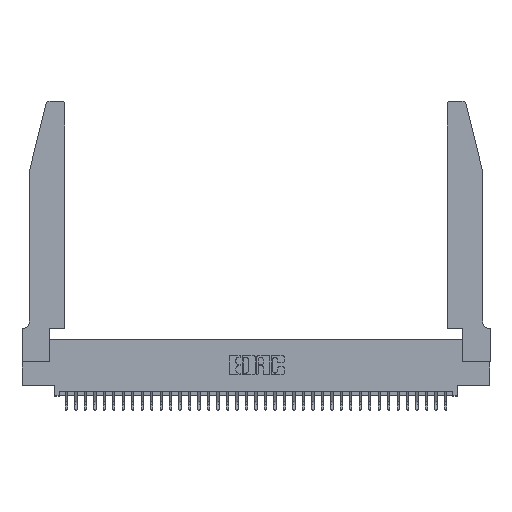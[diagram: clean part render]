
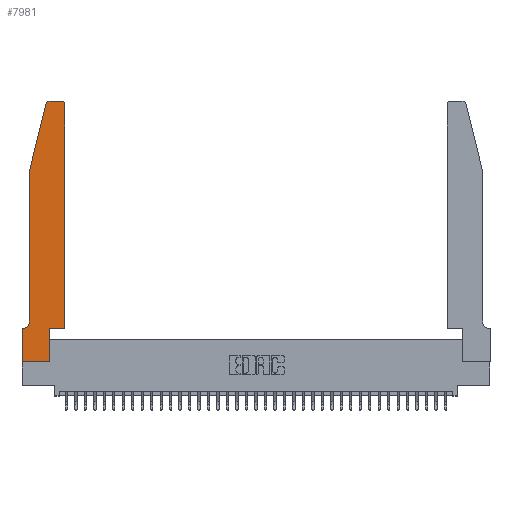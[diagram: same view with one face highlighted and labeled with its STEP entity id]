
A CAD part, top view. The second image highlights one B-rep face of the part: STEP entity #7981.
In plain terms, the highlighted planar face has unit normal (0, 0, 1).
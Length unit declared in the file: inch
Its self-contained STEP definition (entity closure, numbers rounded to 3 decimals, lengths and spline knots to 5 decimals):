
#51 = LINE ( 'NONE', #12348, #7271 ) ;
#1088 = DIRECTION ( 'NONE',  ( 0., -1., 0. ) ) ;
#2117 = EDGE_CURVE ( 'NONE', #23884, #32361, #51, .T. ) ;
#2524 = EDGE_CURVE ( 'NONE', #32361, #19270, #25403, .T. ) ;
#2597 = CARTESIAN_POINT ( 'NONE',  ( 0.4505, 0.35, 0.37 ) ) ;
#3032 = EDGE_CURVE ( 'NONE', #11793, #6742, #24887, .T. ) ;
#3141 = DIRECTION ( 'NONE',  ( -1., 0., 0. ) ) ;
#3197 = LINE ( 'NONE', #21606, #13162 ) ;
#3855 = VECTOR ( 'NONE', #11667, 39.37008 ) ;
#4039 = CARTESIAN_POINT ( 'NONE',  ( 0.284, 2.72, 0.37 ) ) ;
#4614 = VECTOR ( 'NONE', #3141, 39.37008 ) ;
#4789 = DIRECTION ( 'NONE',  ( -1., 0., 0. ) ) ;
#4888 = CARTESIAN_POINT ( 'NONE',  ( 0.284, 2.75, 0.37 ) ) ;
#6269 = ORIENTED_EDGE ( 'NONE', *, *, #2524, .T. ) ;
#6742 = VERTEX_POINT ( 'NONE', #8463 ) ;
#7030 = ORIENTED_EDGE ( 'NONE', *, *, #36220, .T. ) ;
#7140 = VERTEX_POINT ( 'NONE', #4888 ) ;
#7239 = VERTEX_POINT ( 'NONE', #24668 ) ;
#7271 = VECTOR ( 'NONE', #9415, 39.37008 ) ;
#7814 = AXIS2_PLACEMENT_3D ( 'NONE', #26194, #31943, #34428 ) ;
#7981 = ADVANCED_FACE ( 'NONE', ( #32245 ), #13651, .T. ) ;
#8097 = DIRECTION ( 'NONE',  ( 1., 0., 0. ) ) ;
#8406 = EDGE_CURVE ( 'NONE', #20728, #28738, #24589, .T. ) ;
#8463 = CARTESIAN_POINT ( 'NONE',  ( 0.0755, 2., 0.37 ) ) ;
#8531 = VERTEX_POINT ( 'NONE', #32707 ) ;
#9072 = VECTOR ( 'NONE', #34392, 39.37008 ) ;
#9250 = CARTESIAN_POINT ( 'NONE',  ( 0.0755, 2., 0.37 ) ) ;
#9415 = DIRECTION ( 'NONE',  ( 1., 0., 0. ) ) ;
#9711 = AXIS2_PLACEMENT_3D ( 'NONE', #4039, #15444, #15561 ) ;
#11203 = VERTEX_POINT ( 'NONE', #29097 ) ;
#11288 = CIRCLE ( 'NONE', #22662, 0.07 ) ;
#11596 = EDGE_CURVE ( 'NONE', #19270, #11203, #34358, .T. ) ;
#11667 = DIRECTION ( 'NONE',  ( 0., -1., 0. ) ) ;
#11793 = VERTEX_POINT ( 'NONE', #14175 ) ;
#12348 = CARTESIAN_POINT ( 'NONE',  ( 0.4505, 0.35, 0.37 ) ) ;
#12419 = DIRECTION ( 'NONE',  ( 0., 0., -1. ) ) ;
#12429 = EDGE_CURVE ( 'NONE', #8531, #7239, #11288, .T. ) ;
#13155 = CIRCLE ( 'NONE', #9711, 0.03 ) ;
#13162 = VECTOR ( 'NONE', #21114, 39.37008 ) ;
#13651 = PLANE ( 'NONE',  #28623 ) ;
#14175 = CARTESIAN_POINT ( 'NONE',  ( 0.25487, 2.72718, 0.37 ) ) ;
#14633 = CARTESIAN_POINT ( 'NONE',  ( 0.0755, 0.35, 0.37 ) ) ;
#14838 = ORIENTED_EDGE ( 'NONE', *, *, #24880, .T. ) ;
#15444 = DIRECTION ( 'NONE',  ( 0., 0., 1. ) ) ;
#15561 = DIRECTION ( 'NONE',  ( 1., 0., 0. ) ) ;
#16167 = CARTESIAN_POINT ( 'NONE',  ( 0.2865, 0.35, 0.37 ) ) ;
#16580 = DIRECTION ( 'NONE',  ( 0., 0., 1. ) ) ;
#17927 = LINE ( 'NONE', #24937, #26523 ) ;
#18444 = LINE ( 'NONE', #25479, #34599 ) ;
#18454 = ORIENTED_EDGE ( 'NONE', *, *, #11596, .T. ) ;
#18481 = CARTESIAN_POINT ( 'NONE',  ( 0., 0., 0.37 ) ) ;
#19039 = CARTESIAN_POINT ( 'NONE',  ( 0.2865, 0., 0.37 ) ) ;
#19270 = VERTEX_POINT ( 'NONE', #34355 ) ;
#19284 = LINE ( 'NONE', #9250, #3855 ) ;
#19637 = CARTESIAN_POINT ( 'NONE',  ( 0., 0.35, 0.37 ) ) ;
#19934 = VECTOR ( 'NONE', #31995, 39.37008 ) ;
#20680 = ORIENTED_EDGE ( 'NONE', *, *, #35561, .T. ) ;
#20728 = VERTEX_POINT ( 'NONE', #32402 ) ;
#21114 = DIRECTION ( 'NONE',  ( 0., 1., 0. ) ) ;
#21606 = CARTESIAN_POINT ( 'NONE',  ( 0.2865, 0.35, 0.37 ) ) ;
#21758 = ORIENTED_EDGE ( 'NONE', *, *, #28533, .T. ) ;
#22287 = DIRECTION ( 'NONE',  ( 1., 0., 0. ) ) ;
#22321 = ORIENTED_EDGE ( 'NONE', *, *, #2117, .T. ) ;
#22484 = CARTESIAN_POINT ( 'NONE',  ( 0.0755, 2., 0.37 ) ) ;
#22662 = AXIS2_PLACEMENT_3D ( 'NONE', #29158, #12419, #28393 ) ;
#22896 = ORIENTED_EDGE ( 'NONE', *, *, #32350, .T. ) ;
#23884 = VERTEX_POINT ( 'NONE', #16167 ) ;
#24589 = LINE ( 'NONE', #18481, #35830 ) ;
#24668 = CARTESIAN_POINT ( 'NONE',  ( 0.0055, 0.35, 0.37 ) ) ;
#24880 = EDGE_CURVE ( 'NONE', #7239, #20728, #25909, .T. ) ;
#24887 = LINE ( 'NONE', #22484, #19934 ) ;
#24937 = CARTESIAN_POINT ( 'NONE',  ( 0.2605, 2.75, 0.37 ) ) ;
#25403 = LINE ( 'NONE', #2597, #9072 ) ;
#25479 = CARTESIAN_POINT ( 'NONE',  ( 0., 0., 0.37 ) ) ;
#25909 = LINE ( 'NONE', #14633, #4614 ) ;
#26076 = EDGE_LOOP ( 'NONE', ( #33626, #20680, #27676, #21758, #32312, #14838, #26564, #22896, #7030, #22321, #6269, #18454 ) ) ;
#26194 = CARTESIAN_POINT ( 'NONE',  ( 0.4205, 2.72, 0.37 ) ) ;
#26523 = VECTOR ( 'NONE', #4789, 39.37008 ) ;
#26564 = ORIENTED_EDGE ( 'NONE', *, *, #8406, .T. ) ;
#27676 = ORIENTED_EDGE ( 'NONE', *, *, #3032, .T. ) ;
#28393 = DIRECTION ( 'NONE',  ( -1., 0., 0. ) ) ;
#28533 = EDGE_CURVE ( 'NONE', #6742, #8531, #19284, .T. ) ;
#28623 = AXIS2_PLACEMENT_3D ( 'NONE', #19637, #16580, #22287 ) ;
#28738 = VERTEX_POINT ( 'NONE', #29621 ) ;
#29097 = CARTESIAN_POINT ( 'NONE',  ( 0.4205, 2.75, 0.37 ) ) ;
#29158 = CARTESIAN_POINT ( 'NONE',  ( 0.0055, 0.42, 0.37 ) ) ;
#29621 = CARTESIAN_POINT ( 'NONE',  ( 0., 0., 0.37 ) ) ;
#30998 = CARTESIAN_POINT ( 'NONE',  ( 0.4505, 0.35, 0.37 ) ) ;
#31943 = DIRECTION ( 'NONE',  ( 0., 0., 1. ) ) ;
#31995 = DIRECTION ( 'NONE',  ( -0.239, -0.971, 0. ) ) ;
#32245 = FACE_OUTER_BOUND ( 'NONE', #26076, .T. ) ;
#32312 = ORIENTED_EDGE ( 'NONE', *, *, #12429, .T. ) ;
#32350 = EDGE_CURVE ( 'NONE', #28738, #35048, #18444, .T. ) ;
#32361 = VERTEX_POINT ( 'NONE', #30998 ) ;
#32402 = CARTESIAN_POINT ( 'NONE',  ( 0., 0.35, 0.37 ) ) ;
#32707 = CARTESIAN_POINT ( 'NONE',  ( 0.0755, 0.42, 0.37 ) ) ;
#32851 = EDGE_CURVE ( 'NONE', #11203, #7140, #17927, .T. ) ;
#33626 = ORIENTED_EDGE ( 'NONE', *, *, #32851, .T. ) ;
#34355 = CARTESIAN_POINT ( 'NONE',  ( 0.4505, 2.72, 0.37 ) ) ;
#34358 = CIRCLE ( 'NONE', #7814, 0.03 ) ;
#34392 = DIRECTION ( 'NONE',  ( 0., 1., 0. ) ) ;
#34428 = DIRECTION ( 'NONE',  ( 1., 0., 0. ) ) ;
#34599 = VECTOR ( 'NONE', #8097, 39.37008 ) ;
#35048 = VERTEX_POINT ( 'NONE', #19039 ) ;
#35561 = EDGE_CURVE ( 'NONE', #7140, #11793, #13155, .T. ) ;
#35830 = VECTOR ( 'NONE', #1088, 39.37008 ) ;
#36220 = EDGE_CURVE ( 'NONE', #35048, #23884, #3197, .T. ) ;
